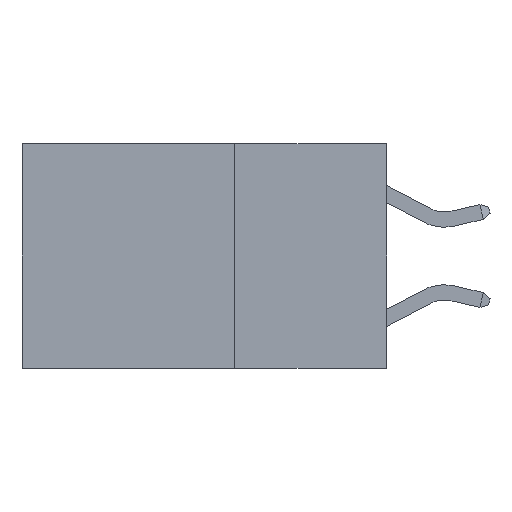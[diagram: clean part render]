
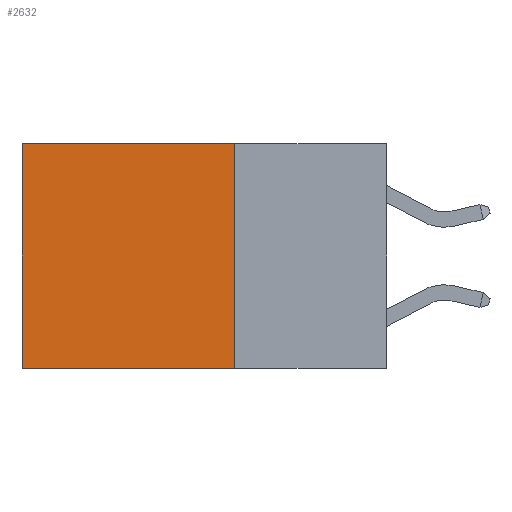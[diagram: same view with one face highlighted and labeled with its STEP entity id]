
A CAD part, left-side view. The second image highlights one B-rep face of the part: STEP entity #2632.
In plain terms, the highlighted planar face has unit normal (-1, 0, 0).
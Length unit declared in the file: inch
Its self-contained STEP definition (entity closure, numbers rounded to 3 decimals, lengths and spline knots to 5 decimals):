
#69 = DIRECTION ( 'NONE',  ( 1., 0., 0. ) ) ;
#429 = EDGE_CURVE ( 'NONE', #2913, #1208, #3024, .T. ) ;
#1005 = EDGE_CURVE ( 'NONE', #1208, #4524, #8375, .T. ) ;
#1128 = CARTESIAN_POINT ( 'NONE',  ( 0.2625, 0.25, 0. ) ) ;
#1208 = VERTEX_POINT ( 'NONE', #1990 ) ;
#1262 = PLANE ( 'NONE',  #6123 ) ;
#1362 = VECTOR ( 'NONE', #6287, 39.37008 ) ;
#1990 = CARTESIAN_POINT ( 'NONE',  ( 0.2625, 0.6, 0. ) ) ;
#2310 = DIRECTION ( 'NONE',  ( 0., 0., -1. ) ) ;
#2632 = ADVANCED_FACE ( 'NONE', ( #10735 ), #1262, .F. ) ;
#2665 = ORIENTED_EDGE ( 'NONE', *, *, #429, .T. ) ;
#2913 = VERTEX_POINT ( 'NONE', #6027 ) ;
#3024 = LINE ( 'NONE', #12627, #5584 ) ;
#3680 = ORIENTED_EDGE ( 'NONE', *, *, #12913, .F. ) ;
#3906 = DIRECTION ( 'NONE',  ( 0., 1., 0. ) ) ;
#4524 = VERTEX_POINT ( 'NONE', #5327 ) ;
#4684 = LINE ( 'NONE', #7076, #1362 ) ;
#5327 = CARTESIAN_POINT ( 'NONE',  ( 0.2625, 0.6, -0.37 ) ) ;
#5335 = ORIENTED_EDGE ( 'NONE', *, *, #6738, .F. ) ;
#5414 = VECTOR ( 'NONE', #2310, 39.37008 ) ;
#5584 = VECTOR ( 'NONE', #3906, 39.37008 ) ;
#5594 = LINE ( 'NONE', #8853, #6939 ) ;
#6027 = CARTESIAN_POINT ( 'NONE',  ( 0.2625, 0.25, 0. ) ) ;
#6123 = AXIS2_PLACEMENT_3D ( 'NONE', #1128, #69, #9821 ) ;
#6287 = DIRECTION ( 'NONE',  ( 0., 0., -1. ) ) ;
#6738 = EDGE_CURVE ( 'NONE', #2913, #11325, #4684, .T. ) ;
#6939 = VECTOR ( 'NONE', #13043, 39.37008 ) ;
#7076 = CARTESIAN_POINT ( 'NONE',  ( 0.2625, 0.25, 0. ) ) ;
#8375 = LINE ( 'NONE', #13654, #5414 ) ;
#8684 = ORIENTED_EDGE ( 'NONE', *, *, #1005, .T. ) ;
#8853 = CARTESIAN_POINT ( 'NONE',  ( 0.2625, 0.25, -0.37 ) ) ;
#9725 = CARTESIAN_POINT ( 'NONE',  ( 0.2625, 0.25, -0.37 ) ) ;
#9821 = DIRECTION ( 'NONE',  ( 0., 0., -1. ) ) ;
#10735 = FACE_OUTER_BOUND ( 'NONE', #10950, .T. ) ;
#10950 = EDGE_LOOP ( 'NONE', ( #8684, #3680, #5335, #2665 ) ) ;
#11325 = VERTEX_POINT ( 'NONE', #9725 ) ;
#12627 = CARTESIAN_POINT ( 'NONE',  ( 0.2625, 0.25, 0. ) ) ;
#12913 = EDGE_CURVE ( 'NONE', #11325, #4524, #5594, .T. ) ;
#13043 = DIRECTION ( 'NONE',  ( 0., 1., 0. ) ) ;
#13654 = CARTESIAN_POINT ( 'NONE',  ( 0.2625, 0.6, 0. ) ) ;
